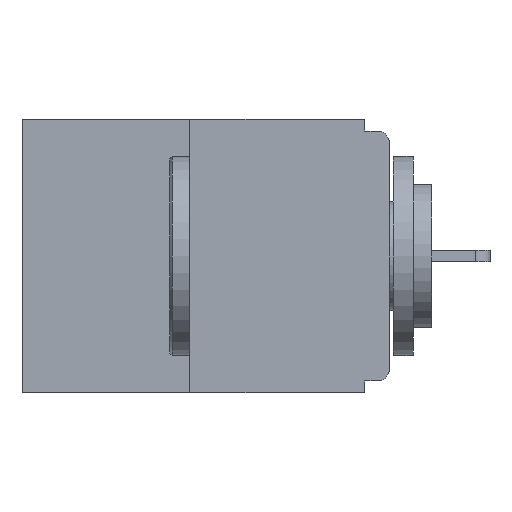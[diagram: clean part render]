
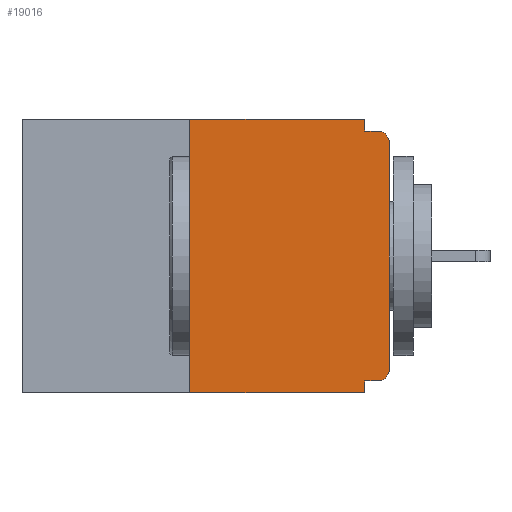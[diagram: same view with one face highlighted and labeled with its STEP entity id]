
A CAD part, left-side view. The second image highlights one B-rep face of the part: STEP entity #19016.
In plain terms, the highlighted planar face has unit normal (-1, 0, 0).
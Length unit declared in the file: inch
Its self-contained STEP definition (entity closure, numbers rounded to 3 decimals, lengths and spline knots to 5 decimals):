
#465 = LINE ( 'NONE', #18486, #21675 ) ;
#666 = ORIENTED_EDGE ( 'NONE', *, *, #7008, .F. ) ;
#830 = EDGE_CURVE ( 'NONE', #13559, #7653, #20177, .T. ) ;
#1086 = VERTEX_POINT ( 'NONE', #3099 ) ;
#1103 = EDGE_CURVE ( 'NONE', #1837, #19891, #10503, .T. ) ;
#1698 = DIRECTION ( 'NONE',  ( 1., 0., 0. ) ) ;
#1721 = DIRECTION ( 'NONE',  ( 0., 0., -1. ) ) ;
#1743 = ORIENTED_EDGE ( 'NONE', *, *, #830, .F. ) ;
#1833 = DIRECTION ( 'NONE',  ( 0., -1., 0. ) ) ;
#1837 = VERTEX_POINT ( 'NONE', #10362 ) ;
#1922 = CARTESIAN_POINT ( 'NONE',  ( 0., 0.031, 0. ) ) ;
#1931 = VERTEX_POINT ( 'NONE', #8828 ) ;
#1943 = DIRECTION ( 'NONE',  ( 0., 0., 1. ) ) ;
#2018 = CIRCLE ( 'NONE', #5265, 0.015 ) ;
#2144 = CIRCLE ( 'NONE', #13760, 0.015 ) ;
#2423 = LINE ( 'NONE', #16498, #11823 ) ;
#2445 = EDGE_CURVE ( 'NONE', #13559, #1931, #5748, .T. ) ;
#2486 = FACE_OUTER_BOUND ( 'NONE', #3937, .T. ) ;
#3023 = CARTESIAN_POINT ( 'NONE',  ( 0., 0., -0.015 ) ) ;
#3099 = CARTESIAN_POINT ( 'NONE',  ( 0., 0., -0.03 ) ) ;
#3937 = EDGE_LOOP ( 'NONE', ( #18526, #1743, #16217, #21094, #21598, #17760, #4907, #6977, #11975, #666 ) ) ;
#4907 = ORIENTED_EDGE ( 'NONE', *, *, #10007, .T. ) ;
#5003 = CARTESIAN_POINT ( 'NONE',  ( 0., 0.46, 0. ) ) ;
#5216 = LINE ( 'NONE', #20947, #14144 ) ;
#5265 = AXIS2_PLACEMENT_3D ( 'NONE', #14865, #14651, #14628 ) ;
#5748 = LINE ( 'NONE', #9978, #19126 ) ;
#5801 = CARTESIAN_POINT ( 'NONE',  ( 0., 0.015, -0.328 ) ) ;
#6036 = CARTESIAN_POINT ( 'NONE',  ( 0., 0.015, -0.015 ) ) ;
#6466 = EDGE_CURVE ( 'NONE', #7653, #19238, #465, .T. ) ;
#6977 = ORIENTED_EDGE ( 'NONE', *, *, #20979, .T. ) ;
#7008 = EDGE_CURVE ( 'NONE', #19238, #1837, #15220, .T. ) ;
#7142 = LINE ( 'NONE', #10276, #15604 ) ;
#7653 = VERTEX_POINT ( 'NONE', #19699 ) ;
#8103 = EDGE_CURVE ( 'NONE', #16199, #21513, #2018, .T. ) ;
#8189 = CARTESIAN_POINT ( 'NONE',  ( 0., 0.25, 0. ) ) ;
#8828 = CARTESIAN_POINT ( 'NONE',  ( 0., 0.031, -0.343 ) ) ;
#8928 = DIRECTION ( 'NONE',  ( 0., 0., 1. ) ) ;
#8943 = CARTESIAN_POINT ( 'NONE',  ( 0., 0.031, 0. ) ) ;
#9824 = DIRECTION ( 'NONE',  ( -1., 0., 0. ) ) ;
#9978 = CARTESIAN_POINT ( 'NONE',  ( 0., 0.46, -0.343 ) ) ;
#10007 = EDGE_CURVE ( 'NONE', #21513, #1086, #7142, .T. ) ;
#10276 = CARTESIAN_POINT ( 'NONE',  ( 0., 0., 0. ) ) ;
#10362 = CARTESIAN_POINT ( 'NONE',  ( 0., 0.031, -0.015 ) ) ;
#10503 = LINE ( 'NONE', #3023, #18898 ) ;
#10714 = VECTOR ( 'NONE', #1721, 39.37008 ) ;
#11090 = EDGE_CURVE ( 'NONE', #14630, #1931, #2423, .T. ) ;
#11561 = CARTESIAN_POINT ( 'NONE',  ( 0., 0.25, -0.343 ) ) ;
#11823 = VECTOR ( 'NONE', #19806, 39.37008 ) ;
#11975 = ORIENTED_EDGE ( 'NONE', *, *, #1103, .F. ) ;
#12355 = VECTOR ( 'NONE', #8928, 39.37008 ) ;
#12658 = DIRECTION ( 'NONE',  ( 0., 1., 0. ) ) ;
#13451 = DIRECTION ( 'NONE',  ( 0., 0., -1. ) ) ;
#13559 = VERTEX_POINT ( 'NONE', #11561 ) ;
#13760 = AXIS2_PLACEMENT_3D ( 'NONE', #19840, #9824, #21491 ) ;
#13813 = DIRECTION ( 'NONE',  ( 0., -1., 0. ) ) ;
#14144 = VECTOR ( 'NONE', #12658, 39.37008 ) ;
#14628 = DIRECTION ( 'NONE',  ( 0., 0., -1. ) ) ;
#14630 = VERTEX_POINT ( 'NONE', #15009 ) ;
#14651 = DIRECTION ( 'NONE',  ( -1., 0., 0. ) ) ;
#14865 = CARTESIAN_POINT ( 'NONE',  ( 0., 0.015, -0.313 ) ) ;
#15009 = CARTESIAN_POINT ( 'NONE',  ( 0., 0.031, -0.328 ) ) ;
#15220 = LINE ( 'NONE', #1922, #10714 ) ;
#15604 = VECTOR ( 'NONE', #1943, 39.37008 ) ;
#15657 = EDGE_CURVE ( 'NONE', #16199, #14630, #5216, .T. ) ;
#16199 = VERTEX_POINT ( 'NONE', #5801 ) ;
#16217 = ORIENTED_EDGE ( 'NONE', *, *, #2445, .T. ) ;
#16498 = CARTESIAN_POINT ( 'NONE',  ( 0., 0.031, -0.343 ) ) ;
#17760 = ORIENTED_EDGE ( 'NONE', *, *, #8103, .T. ) ;
#17781 = AXIS2_PLACEMENT_3D ( 'NONE', #5003, #1698, #13451 ) ;
#18418 = PLANE ( 'NONE',  #17781 ) ;
#18486 = CARTESIAN_POINT ( 'NONE',  ( 0., 0.46, 0. ) ) ;
#18524 = DIRECTION ( 'NONE',  ( 0., -1., 0. ) ) ;
#18526 = ORIENTED_EDGE ( 'NONE', *, *, #6466, .F. ) ;
#18898 = VECTOR ( 'NONE', #1833, 39.37008 ) ;
#19016 = ADVANCED_FACE ( 'NONE', ( #2486 ), #18418, .F. ) ;
#19126 = VECTOR ( 'NONE', #13813, 39.37008 ) ;
#19238 = VERTEX_POINT ( 'NONE', #8943 ) ;
#19699 = CARTESIAN_POINT ( 'NONE',  ( 0., 0.25, 0. ) ) ;
#19806 = DIRECTION ( 'NONE',  ( 0., 0., -1. ) ) ;
#19840 = CARTESIAN_POINT ( 'NONE',  ( 0., 0.015, -0.03 ) ) ;
#19891 = VERTEX_POINT ( 'NONE', #6036 ) ;
#20177 = LINE ( 'NONE', #8189, #12355 ) ;
#20947 = CARTESIAN_POINT ( 'NONE',  ( 0., 0., -0.328 ) ) ;
#20979 = EDGE_CURVE ( 'NONE', #1086, #19891, #2144, .T. ) ;
#21094 = ORIENTED_EDGE ( 'NONE', *, *, #11090, .F. ) ;
#21330 = CARTESIAN_POINT ( 'NONE',  ( 0., 0., -0.313 ) ) ;
#21491 = DIRECTION ( 'NONE',  ( 0., 0., -1. ) ) ;
#21513 = VERTEX_POINT ( 'NONE', #21330 ) ;
#21598 = ORIENTED_EDGE ( 'NONE', *, *, #15657, .F. ) ;
#21675 = VECTOR ( 'NONE', #18524, 39.37008 ) ;
